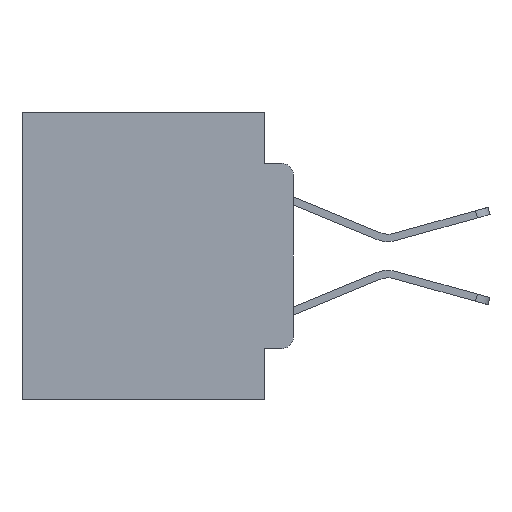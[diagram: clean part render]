
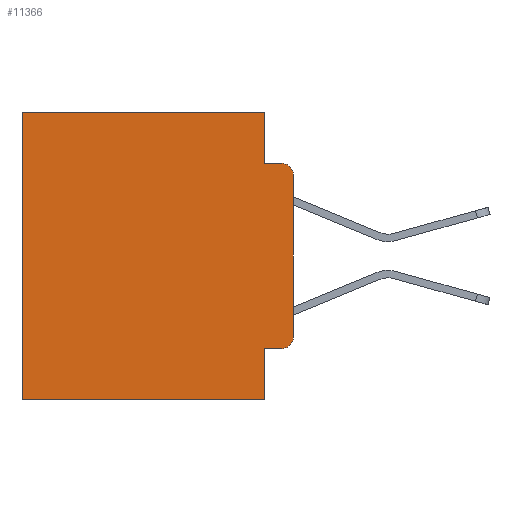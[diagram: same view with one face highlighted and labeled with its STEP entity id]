
A CAD part, left-side view. The second image highlights one B-rep face of the part: STEP entity #11366.
In plain terms, the highlighted planar face has unit normal (-1, 0, 0).
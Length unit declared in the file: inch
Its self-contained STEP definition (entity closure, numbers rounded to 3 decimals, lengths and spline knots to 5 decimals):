
#754 = PLANE ( 'NONE',  #26180 ) ;
#871 = ORIENTED_EDGE ( 'NONE', *, *, #24095, .F. ) ;
#1485 = LINE ( 'NONE', #18703, #23796 ) ;
#1857 = EDGE_CURVE ( 'NONE', #5123, #11772, #1485, .T. ) ;
#2192 = AXIS2_PLACEMENT_3D ( 'NONE', #21358, #15189, #23718 ) ;
#3014 = DIRECTION ( 'NONE',  ( 0., 0., -1. ) ) ;
#3122 = DIRECTION ( 'NONE',  ( 0., 1., 0. ) ) ;
#3488 = LINE ( 'NONE', #12784, #13624 ) ;
#3661 = CARTESIAN_POINT ( 'NONE',  ( 0.298, 0.473, 0. ) ) ;
#4393 = ORIENTED_EDGE ( 'NONE', *, *, #27045, .T. ) ;
#4434 = EDGE_CURVE ( 'NONE', #8233, #7874, #26310, .T. ) ;
#4622 = CARTESIAN_POINT ( 'NONE',  ( 0.298, 0.051, 0. ) ) ;
#4644 = EDGE_CURVE ( 'NONE', #5685, #18386, #25318, .T. ) ;
#4903 = CARTESIAN_POINT ( 'NONE',  ( 0.298, 0.051, -0.4115 ) ) ;
#5123 = VERTEX_POINT ( 'NONE', #24035 ) ;
#5685 = VERTEX_POINT ( 'NONE', #4622 ) ;
#5777 = DIRECTION ( 'NONE',  ( 0., 0., -1. ) ) ;
#6823 = DIRECTION ( 'NONE',  ( 1., 0., 0. ) ) ;
#6967 = ORIENTED_EDGE ( 'NONE', *, *, #27049, .T. ) ;
#7353 = CARTESIAN_POINT ( 'NONE',  ( 0.298, 0., 0. ) ) ;
#7425 = CARTESIAN_POINT ( 'NONE',  ( 0.298, 0.02, -0.1085 ) ) ;
#7874 = VERTEX_POINT ( 'NONE', #10797 ) ;
#7932 = CARTESIAN_POINT ( 'NONE',  ( 0.298, 0., -0.5 ) ) ;
#8003 = LINE ( 'NONE', #23452, #12066 ) ;
#8050 = VECTOR ( 'NONE', #13133, 39.37008 ) ;
#8233 = VERTEX_POINT ( 'NONE', #21962 ) ;
#9643 = CIRCLE ( 'NONE', #11607, 0.02 ) ;
#10686 = CARTESIAN_POINT ( 'NONE',  ( 0.298, 0.02, -0.0885 ) ) ;
#10707 = EDGE_CURVE ( 'NONE', #18386, #25465, #25189, .T. ) ;
#10797 = CARTESIAN_POINT ( 'NONE',  ( 0.298, 0.473, -0.5 ) ) ;
#10928 = CIRCLE ( 'NONE', #2192, 0.02 ) ;
#11091 = VERTEX_POINT ( 'NONE', #3661 ) ;
#11334 = CARTESIAN_POINT ( 'NONE',  ( 0.298, 0.02, -0.4115 ) ) ;
#11366 = ADVANCED_FACE ( 'NONE', ( #23811 ), #754, .F. ) ;
#11607 = AXIS2_PLACEMENT_3D ( 'NONE', #7425, #15915, #3014 ) ;
#11772 = VERTEX_POINT ( 'NONE', #17023 ) ;
#12009 = ORIENTED_EDGE ( 'NONE', *, *, #14385, .T. ) ;
#12066 = VECTOR ( 'NONE', #17084, 39.37008 ) ;
#12784 = CARTESIAN_POINT ( 'NONE',  ( 0.298, 0.051, -0.4115 ) ) ;
#13133 = DIRECTION ( 'NONE',  ( 0., 0., -1. ) ) ;
#13624 = VECTOR ( 'NONE', #26072, 39.37008 ) ;
#14385 = EDGE_CURVE ( 'NONE', #11091, #7874, #8003, .T. ) ;
#15124 = LINE ( 'NONE', #25007, #22228 ) ;
#15189 = DIRECTION ( 'NONE',  ( -1., 0., 0. ) ) ;
#15246 = ORIENTED_EDGE ( 'NONE', *, *, #1857, .F. ) ;
#15319 = ORIENTED_EDGE ( 'NONE', *, *, #4434, .F. ) ;
#15485 = DIRECTION ( 'NONE',  ( 0., 0., -1. ) ) ;
#15915 = DIRECTION ( 'NONE',  ( -1., 0., 0. ) ) ;
#16291 = LINE ( 'NONE', #7353, #25758 ) ;
#16769 = ORIENTED_EDGE ( 'NONE', *, *, #25779, .T. ) ;
#16790 = DIRECTION ( 'NONE',  ( 0., -1., 0. ) ) ;
#17023 = CARTESIAN_POINT ( 'NONE',  ( 0.298, 0., -0.3915 ) ) ;
#17084 = DIRECTION ( 'NONE',  ( 0., 0., -1. ) ) ;
#17424 = CARTESIAN_POINT ( 'NONE',  ( 0.298, 0.051, 0. ) ) ;
#17937 = VERTEX_POINT ( 'NONE', #11334 ) ;
#18067 = VECTOR ( 'NONE', #16790, 39.37008 ) ;
#18386 = VERTEX_POINT ( 'NONE', #26114 ) ;
#18703 = CARTESIAN_POINT ( 'NONE',  ( 0.298, 0., 0. ) ) ;
#19890 = VERTEX_POINT ( 'NONE', #4903 ) ;
#20831 = DIRECTION ( 'NONE',  ( 0., 0., -1. ) ) ;
#21051 = CARTESIAN_POINT ( 'NONE',  ( 0.298, 0.051, -0.0885 ) ) ;
#21358 = CARTESIAN_POINT ( 'NONE',  ( 0.298, 0.02, -0.3915 ) ) ;
#21595 = VECTOR ( 'NONE', #23047, 39.37008 ) ;
#21962 = CARTESIAN_POINT ( 'NONE',  ( 0.298, 0.051, -0.5 ) ) ;
#22228 = VECTOR ( 'NONE', #20831, 39.37008 ) ;
#22605 = ORIENTED_EDGE ( 'NONE', *, *, #27377, .T. ) ;
#22979 = EDGE_LOOP ( 'NONE', ( #15246, #16769, #27443, #27410, #22605, #12009, #15319, #871, #6967, #4393 ) ) ;
#23047 = DIRECTION ( 'NONE',  ( 0., 1., 0. ) ) ;
#23452 = CARTESIAN_POINT ( 'NONE',  ( 0.298, 0.473, 0. ) ) ;
#23718 = DIRECTION ( 'NONE',  ( 0., 0., -1. ) ) ;
#23796 = VECTOR ( 'NONE', #5777, 39.37008 ) ;
#23811 = FACE_OUTER_BOUND ( 'NONE', #22979, .T. ) ;
#24035 = CARTESIAN_POINT ( 'NONE',  ( 0.298, 0., -0.1085 ) ) ;
#24095 = EDGE_CURVE ( 'NONE', #19890, #8233, #15124, .T. ) ;
#25007 = CARTESIAN_POINT ( 'NONE',  ( 0.298, 0.051, 0. ) ) ;
#25189 = LINE ( 'NONE', #21051, #18067 ) ;
#25318 = LINE ( 'NONE', #17424, #8050 ) ;
#25465 = VERTEX_POINT ( 'NONE', #10686 ) ;
#25758 = VECTOR ( 'NONE', #3122, 39.37008 ) ;
#25779 = EDGE_CURVE ( 'NONE', #5123, #25465, #9643, .T. ) ;
#26072 = DIRECTION ( 'NONE',  ( 0., -1., 0. ) ) ;
#26114 = CARTESIAN_POINT ( 'NONE',  ( 0.298, 0.051, -0.0885 ) ) ;
#26180 = AXIS2_PLACEMENT_3D ( 'NONE', #26269, #6823, #15485 ) ;
#26269 = CARTESIAN_POINT ( 'NONE',  ( 0.298, 0., 0. ) ) ;
#26310 = LINE ( 'NONE', #7932, #21595 ) ;
#27045 = EDGE_CURVE ( 'NONE', #17937, #11772, #10928, .T. ) ;
#27049 = EDGE_CURVE ( 'NONE', #19890, #17937, #3488, .T. ) ;
#27377 = EDGE_CURVE ( 'NONE', #5685, #11091, #16291, .T. ) ;
#27410 = ORIENTED_EDGE ( 'NONE', *, *, #4644, .F. ) ;
#27443 = ORIENTED_EDGE ( 'NONE', *, *, #10707, .F. ) ;
